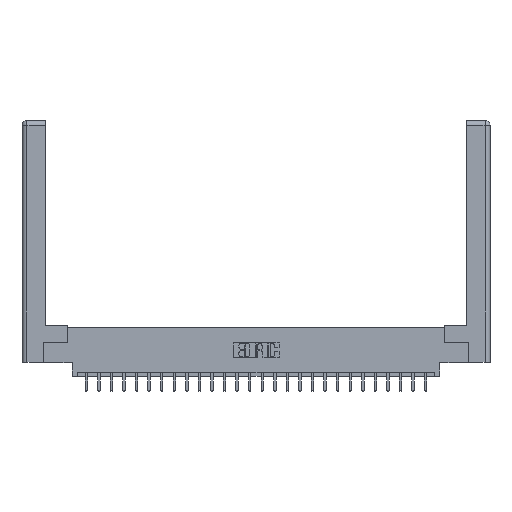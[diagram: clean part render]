
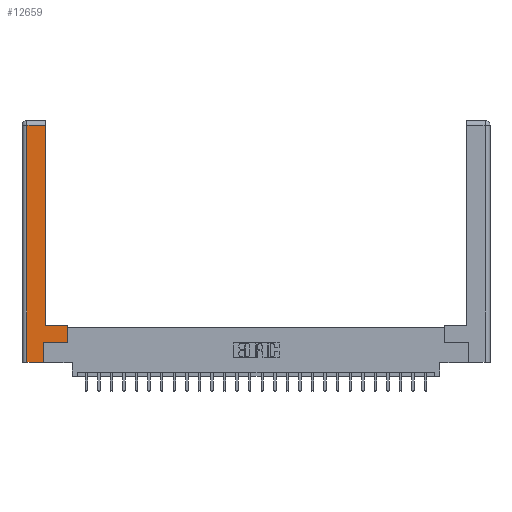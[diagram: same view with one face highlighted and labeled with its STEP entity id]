
A CAD part, top view. The second image highlights one B-rep face of the part: STEP entity #12659.
In plain terms, the highlighted planar face has unit normal (0, 0, 1).
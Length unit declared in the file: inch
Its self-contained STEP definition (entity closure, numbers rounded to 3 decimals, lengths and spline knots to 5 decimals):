
#369 = CARTESIAN_POINT ( 'NONE',  ( 0.0615, 0., 0. ) ) ;
#455 = VECTOR ( 'NONE', #4949, 39.37008 ) ;
#1127 = ORIENTED_EDGE ( 'NONE', *, *, #11388, .T. ) ;
#1392 = AXIS2_PLACEMENT_3D ( 'NONE', #5089, #4091, #14927 ) ;
#1494 = DIRECTION ( 'NONE',  ( 0., -1., 0. ) ) ;
#2501 = LINE ( 'NONE', #9927, #15538 ) ;
#2597 = VERTEX_POINT ( 'NONE', #4191 ) ;
#2757 = VERTEX_POINT ( 'NONE', #6318 ) ;
#2889 = ORIENTED_EDGE ( 'NONE', *, *, #11992, .T. ) ;
#4091 = DIRECTION ( 'NONE',  ( 0., 0., -1. ) ) ;
#4191 = CARTESIAN_POINT ( 'NONE',  ( 0.295, 2.94, 0. ) ) ;
#4477 = ORIENTED_EDGE ( 'NONE', *, *, #6248, .T. ) ;
#4949 = DIRECTION ( 'NONE',  ( 0., 1., 0. ) ) ;
#5089 = CARTESIAN_POINT ( 'NONE',  ( 0., 0., 0. ) ) ;
#5463 = LINE ( 'NONE', #25977, #21114 ) ;
#6099 = ORIENTED_EDGE ( 'NONE', *, *, #26096, .T. ) ;
#6248 = EDGE_CURVE ( 'NONE', #17807, #2597, #15168, .T. ) ;
#6318 = CARTESIAN_POINT ( 'NONE',  ( 0.265, 0., 0. ) ) ;
#6979 = DIRECTION ( 'NONE',  ( 1., 0., 0. ) ) ;
#7058 = CARTESIAN_POINT ( 'NONE',  ( 0.295, 0.45, 0. ) ) ;
#7357 = FACE_OUTER_BOUND ( 'NONE', #11299, .T. ) ;
#7977 = LINE ( 'NONE', #19182, #21344 ) ;
#8270 = ORIENTED_EDGE ( 'NONE', *, *, #16183, .T. ) ;
#8733 = VERTEX_POINT ( 'NONE', #12113 ) ;
#8923 = DIRECTION ( 'NONE',  ( 0., 1., 0. ) ) ;
#9927 = CARTESIAN_POINT ( 'NONE',  ( 0.265, 0.245, 0. ) ) ;
#10616 = LINE ( 'NONE', #19742, #19494 ) ;
#10624 = VECTOR ( 'NONE', #19676, 39.37008 ) ;
#10767 = CARTESIAN_POINT ( 'NONE',  ( 0.565, 0.245, 0. ) ) ;
#11299 = EDGE_LOOP ( 'NONE', ( #4477, #19921, #11877, #6099, #1127, #2889, #22828, #8270 ) ) ;
#11388 = EDGE_CURVE ( 'NONE', #2757, #8733, #2501, .T. ) ;
#11687 = VECTOR ( 'NONE', #8923, 39.37008 ) ;
#11877 = ORIENTED_EDGE ( 'NONE', *, *, #21849, .T. ) ;
#11992 = EDGE_CURVE ( 'NONE', #8733, #13866, #5463, .T. ) ;
#12113 = CARTESIAN_POINT ( 'NONE',  ( 0.265, 0.245, 0. ) ) ;
#12201 = VERTEX_POINT ( 'NONE', #369 ) ;
#12659 = ADVANCED_FACE ( 'NONE', ( #7357 ), #15773, .F. ) ;
#13072 = CARTESIAN_POINT ( 'NONE',  ( 0.0615, 2.94, 0. ) ) ;
#13684 = DIRECTION ( 'NONE',  ( 1., 0., 0. ) ) ;
#13866 = VERTEX_POINT ( 'NONE', #10767 ) ;
#14107 = CARTESIAN_POINT ( 'NONE',  ( 0.565, 0.45, 0. ) ) ;
#14927 = DIRECTION ( 'NONE',  ( -1., 0., 0. ) ) ;
#15168 = LINE ( 'NONE', #17079, #11687 ) ;
#15538 = VECTOR ( 'NONE', #20175, 39.37008 ) ;
#15773 = PLANE ( 'NONE',  #1392 ) ;
#16183 = EDGE_CURVE ( 'NONE', #21893, #17807, #17620, .T. ) ;
#16376 = EDGE_CURVE ( 'NONE', #13866, #21893, #20543, .T. ) ;
#17079 = CARTESIAN_POINT ( 'NONE',  ( 0.295, 3., 0. ) ) ;
#17098 = CARTESIAN_POINT ( 'NONE',  ( 0.295, 0.45, 0. ) ) ;
#17620 = LINE ( 'NONE', #7058, #26326 ) ;
#17807 = VERTEX_POINT ( 'NONE', #17098 ) ;
#18466 = VERTEX_POINT ( 'NONE', #13072 ) ;
#19182 = CARTESIAN_POINT ( 'NONE',  ( 0.265, 0., 0. ) ) ;
#19494 = VECTOR ( 'NONE', #1494, 39.37008 ) ;
#19676 = DIRECTION ( 'NONE',  ( -1., 0., 0. ) ) ;
#19742 = CARTESIAN_POINT ( 'NONE',  ( 0.0615, 0., 0. ) ) ;
#19921 = ORIENTED_EDGE ( 'NONE', *, *, #22559, .T. ) ;
#20175 = DIRECTION ( 'NONE',  ( 0., 1., 0. ) ) ;
#20543 = LINE ( 'NONE', #14107, #455 ) ;
#21114 = VECTOR ( 'NONE', #13684, 39.37008 ) ;
#21344 = VECTOR ( 'NONE', #6979, 39.37008 ) ;
#21849 = EDGE_CURVE ( 'NONE', #18466, #12201, #10616, .T. ) ;
#21893 = VERTEX_POINT ( 'NONE', #22112 ) ;
#22112 = CARTESIAN_POINT ( 'NONE',  ( 0.565, 0.45, 0. ) ) ;
#22559 = EDGE_CURVE ( 'NONE', #2597, #18466, #23057, .T. ) ;
#22828 = ORIENTED_EDGE ( 'NONE', *, *, #16376, .T. ) ;
#23057 = LINE ( 'NONE', #25704, #10624 ) ;
#23394 = DIRECTION ( 'NONE',  ( -1., 0., 0. ) ) ;
#25704 = CARTESIAN_POINT ( 'NONE',  ( 0.0615, 2.94, 0. ) ) ;
#25977 = CARTESIAN_POINT ( 'NONE',  ( 0.565, 0.245, 0. ) ) ;
#26096 = EDGE_CURVE ( 'NONE', #12201, #2757, #7977, .T. ) ;
#26326 = VECTOR ( 'NONE', #23394, 39.37008 ) ;
